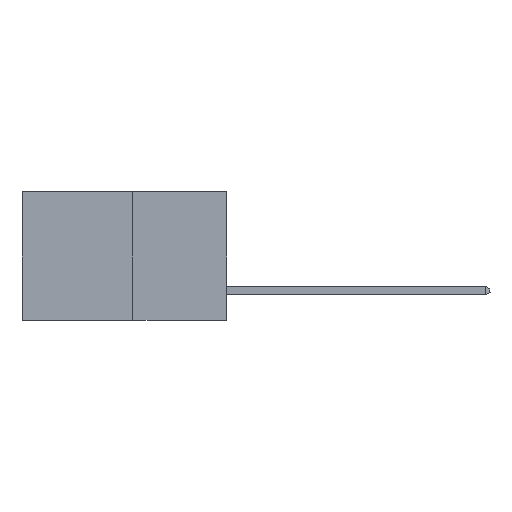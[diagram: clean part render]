
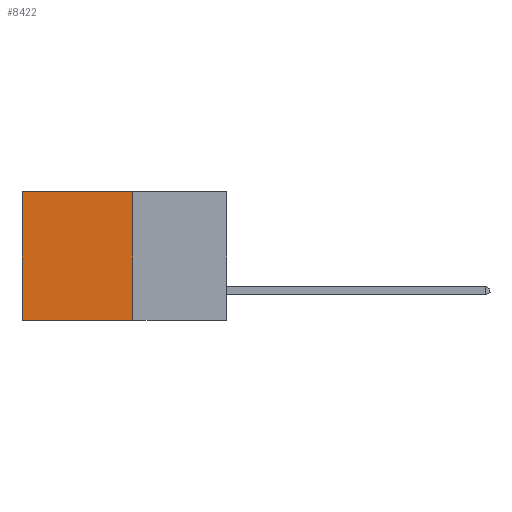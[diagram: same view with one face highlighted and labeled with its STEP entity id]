
A CAD part, left-side view. The second image highlights one B-rep face of the part: STEP entity #8422.
In plain terms, the highlighted planar face has unit normal (-1, 0, 0).
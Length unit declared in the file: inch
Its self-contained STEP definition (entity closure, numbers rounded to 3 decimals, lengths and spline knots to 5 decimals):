
#118 = VECTOR ( 'NONE', #2061, 39.37008 ) ;
#636 = VERTEX_POINT ( 'NONE', #20151 ) ;
#706 = EDGE_CURVE ( 'NONE', #636, #7762, #4608, .T. ) ;
#784 = FACE_OUTER_BOUND ( 'NONE', #8677, .T. ) ;
#796 = CARTESIAN_POINT ( 'NONE',  ( 0.277, 0.59, -0.37 ) ) ;
#2061 = DIRECTION ( 'NONE',  ( 0., 1., 0. ) ) ;
#2941 = LINE ( 'NONE', #13731, #19937 ) ;
#3494 = CARTESIAN_POINT ( 'NONE',  ( 0.277, 0.27, 0. ) ) ;
#3689 = CARTESIAN_POINT ( 'NONE',  ( 0.277, 0.27, -0.37 ) ) ;
#4608 = LINE ( 'NONE', #3689, #118 ) ;
#4753 = VECTOR ( 'NONE', #14074, 39.37008 ) ;
#5516 = CARTESIAN_POINT ( 'NONE',  ( 0.277, 0.59, 0. ) ) ;
#5957 = CARTESIAN_POINT ( 'NONE',  ( 0.277, 0.59, -0.37 ) ) ;
#6089 = VERTEX_POINT ( 'NONE', #5516 ) ;
#6209 = ORIENTED_EDGE ( 'NONE', *, *, #16080, .T. ) ;
#7031 = EDGE_CURVE ( 'NONE', #12014, #6089, #2941, .T. ) ;
#7762 = VERTEX_POINT ( 'NONE', #5957 ) ;
#8422 = ADVANCED_FACE ( 'NONE', ( #784 ), #13482, .F. ) ;
#8677 = EDGE_LOOP ( 'NONE', ( #6209, #13951, #21352, #13745 ) ) ;
#9301 = AXIS2_PLACEMENT_3D ( 'NONE', #12699, #12019, #11853 ) ;
#9734 = LINE ( 'NONE', #796, #4753 ) ;
#11853 = DIRECTION ( 'NONE',  ( 0., 0., -1. ) ) ;
#11963 = LINE ( 'NONE', #19257, #16292 ) ;
#12014 = VERTEX_POINT ( 'NONE', #3494 ) ;
#12019 = DIRECTION ( 'NONE',  ( 1., 0., 0. ) ) ;
#12699 = CARTESIAN_POINT ( 'NONE',  ( 0.277, 0.27, -0.37 ) ) ;
#13482 = PLANE ( 'NONE',  #9301 ) ;
#13690 = DIRECTION ( 'NONE',  ( 0., 1., 0. ) ) ;
#13731 = CARTESIAN_POINT ( 'NONE',  ( 0.277, 0.27, 0. ) ) ;
#13745 = ORIENTED_EDGE ( 'NONE', *, *, #7031, .T. ) ;
#13951 = ORIENTED_EDGE ( 'NONE', *, *, #706, .F. ) ;
#14074 = DIRECTION ( 'NONE',  ( 0., 0., -1. ) ) ;
#16059 = DIRECTION ( 'NONE',  ( 0., 0., -1. ) ) ;
#16080 = EDGE_CURVE ( 'NONE', #6089, #7762, #9734, .T. ) ;
#16292 = VECTOR ( 'NONE', #16059, 39.37008 ) ;
#18098 = EDGE_CURVE ( 'NONE', #12014, #636, #11963, .T. ) ;
#19257 = CARTESIAN_POINT ( 'NONE',  ( 0.277, 0.27, -0.37 ) ) ;
#19937 = VECTOR ( 'NONE', #13690, 39.37008 ) ;
#20151 = CARTESIAN_POINT ( 'NONE',  ( 0.277, 0.27, -0.37 ) ) ;
#21352 = ORIENTED_EDGE ( 'NONE', *, *, #18098, .F. ) ;
